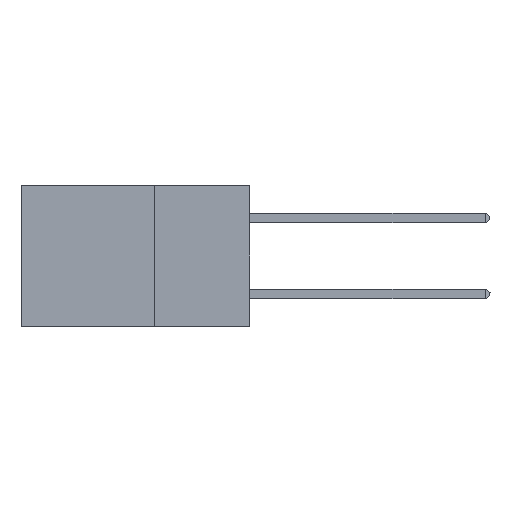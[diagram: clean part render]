
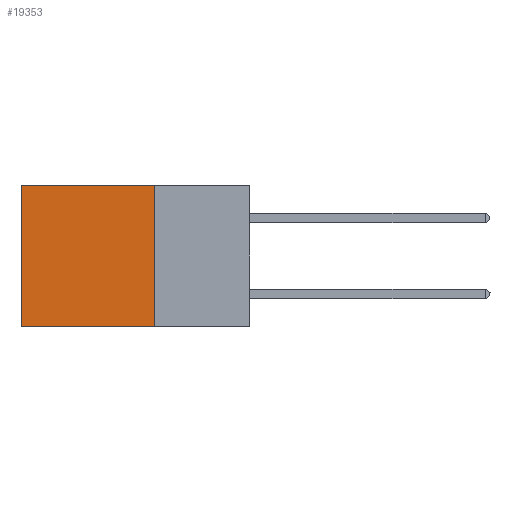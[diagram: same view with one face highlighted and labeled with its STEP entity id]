
A CAD part, left-side view. The second image highlights one B-rep face of the part: STEP entity #19353.
In plain terms, the highlighted planar face has unit normal (-1, 0, 0).
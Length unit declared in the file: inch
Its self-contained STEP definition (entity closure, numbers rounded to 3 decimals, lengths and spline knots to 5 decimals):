
#25 = DIRECTION ( 'NONE',  ( 0., 1., 0. ) ) ;
#801 = VECTOR ( 'NONE', #25, 39.37008 ) ;
#1842 = LINE ( 'NONE', #26433, #801 ) ;
#3104 = CARTESIAN_POINT ( 'NONE',  ( 0.2875, 0.6, -0.37 ) ) ;
#3333 = DIRECTION ( 'NONE',  ( 1., 0., 0. ) ) ;
#4565 = VERTEX_POINT ( 'NONE', #6908 ) ;
#5229 = CARTESIAN_POINT ( 'NONE',  ( 0.2875, 0.6, 0. ) ) ;
#5332 = CARTESIAN_POINT ( 'NONE',  ( 0.2875, 0.25, 0. ) ) ;
#5449 = CARTESIAN_POINT ( 'NONE',  ( 0.2875, 0.25, 0. ) ) ;
#5608 = LINE ( 'NONE', #5449, #10427 ) ;
#6908 = CARTESIAN_POINT ( 'NONE',  ( 0.2875, 0.6, 0. ) ) ;
#8138 = VERTEX_POINT ( 'NONE', #3104 ) ;
#9680 = EDGE_CURVE ( 'NONE', #13615, #20925, #22424, .T. ) ;
#10427 = VECTOR ( 'NONE', #27101, 39.37008 ) ;
#11281 = ORIENTED_EDGE ( 'NONE', *, *, #26252, .T. ) ;
#12003 = PLANE ( 'NONE',  #14218 ) ;
#12413 = DIRECTION ( 'NONE',  ( 0., 0., -1. ) ) ;
#12580 = ORIENTED_EDGE ( 'NONE', *, *, #14777, .F. ) ;
#13615 = VERTEX_POINT ( 'NONE', #19000 ) ;
#13797 = CARTESIAN_POINT ( 'NONE',  ( 0.2875, 0.25, -0.37 ) ) ;
#14124 = VECTOR ( 'NONE', #22660, 39.37008 ) ;
#14218 = AXIS2_PLACEMENT_3D ( 'NONE', #5332, #3333, #18686 ) ;
#14699 = EDGE_CURVE ( 'NONE', #13615, #4565, #5608, .T. ) ;
#14777 = EDGE_CURVE ( 'NONE', #20925, #8138, #1842, .T. ) ;
#17243 = FACE_OUTER_BOUND ( 'NONE', #26882, .T. ) ;
#18686 = DIRECTION ( 'NONE',  ( 0., 0., -1. ) ) ;
#19000 = CARTESIAN_POINT ( 'NONE',  ( 0.2875, 0.25, 0. ) ) ;
#19353 = ADVANCED_FACE ( 'NONE', ( #17243 ), #12003, .F. ) ;
#20925 = VERTEX_POINT ( 'NONE', #13797 ) ;
#22033 = LINE ( 'NONE', #5229, #14124 ) ;
#22424 = LINE ( 'NONE', #23540, #25182 ) ;
#22660 = DIRECTION ( 'NONE',  ( 0., 0., -1. ) ) ;
#23540 = CARTESIAN_POINT ( 'NONE',  ( 0.2875, 0.25, 0. ) ) ;
#24089 = ORIENTED_EDGE ( 'NONE', *, *, #9680, .F. ) ;
#25103 = ORIENTED_EDGE ( 'NONE', *, *, #14699, .T. ) ;
#25182 = VECTOR ( 'NONE', #12413, 39.37008 ) ;
#26252 = EDGE_CURVE ( 'NONE', #4565, #8138, #22033, .T. ) ;
#26433 = CARTESIAN_POINT ( 'NONE',  ( 0.2875, 0.25, -0.37 ) ) ;
#26882 = EDGE_LOOP ( 'NONE', ( #11281, #12580, #24089, #25103 ) ) ;
#27101 = DIRECTION ( 'NONE',  ( 0., 1., 0. ) ) ;
